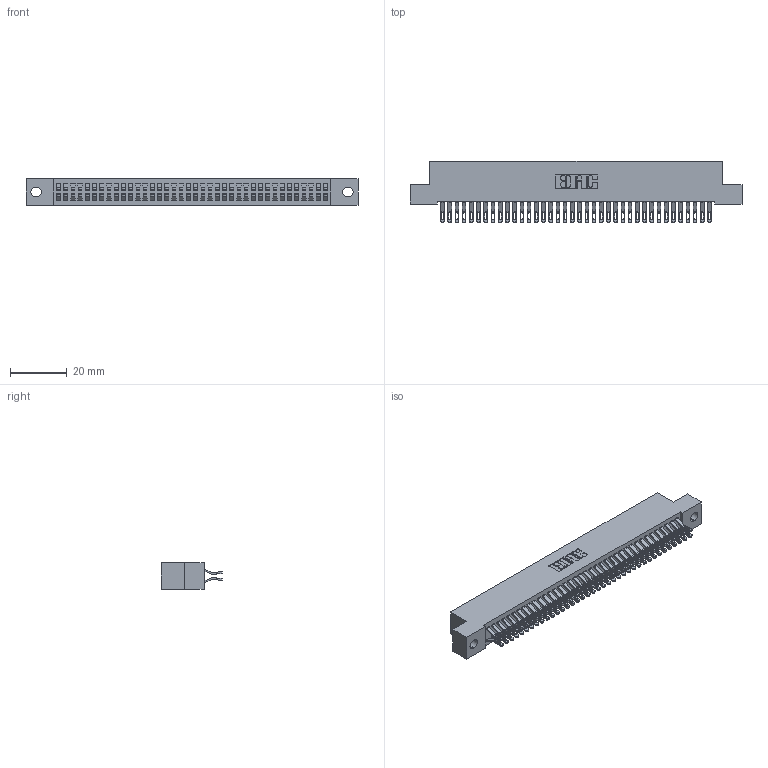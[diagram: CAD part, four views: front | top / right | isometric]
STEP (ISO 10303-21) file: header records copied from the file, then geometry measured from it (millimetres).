
FILE_DESCRIPTION (( 'STEP AP203' ), '1' );
FILE_NAME ('342-076-555-202.STEP', '2019-10-04T10:49:47', ( '' ), ( '' ), 'SwSTEP 2.0', 'SolidWorks 2016', '' );
FILE_SCHEMA (( 'CONFIG_CONTROL_DESIGN' ));
Length unit declared in the file: inch
Products named in the file (3): 342 Part_.128 Slot; 345-292-001_555 Tail; 342-076-555-202
Assembly tree (77 placements, depth 2):
  342-076-555-202
    342 Part_.128 Slot
    345-292-001_555 Tail  x76
Bounding box: 116.84 x 21.47 x 9.4 mm (x, y, z)
Volume: 10638.2 mm3; surface area: 17712.6 mm2
Topology: 77 solids, 77 shells, 4522 faces, 14219 edges, 9478 vertices
Faces by surface type: plane 2654, cylinder 1868
Entity records: 25293 total; most frequent: CARTESIAN_POINT 4232, ORIENTED_EDGE 4138, DIRECTION 3593, EDGE_CURVE 2069, VECTOR 1921, LINE 1921, VERTEX_POINT 1378, AXIS2_PLACEMENT_3D 836
